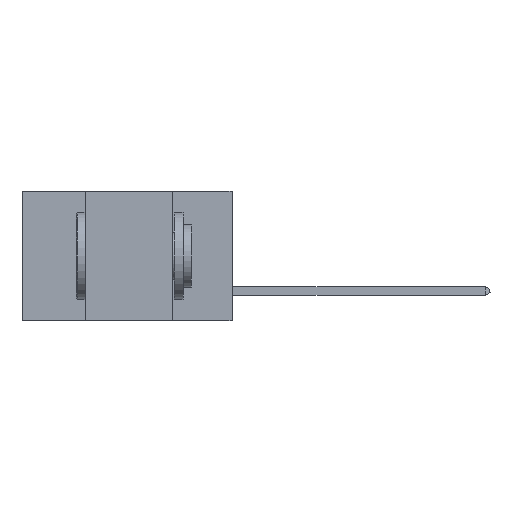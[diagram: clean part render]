
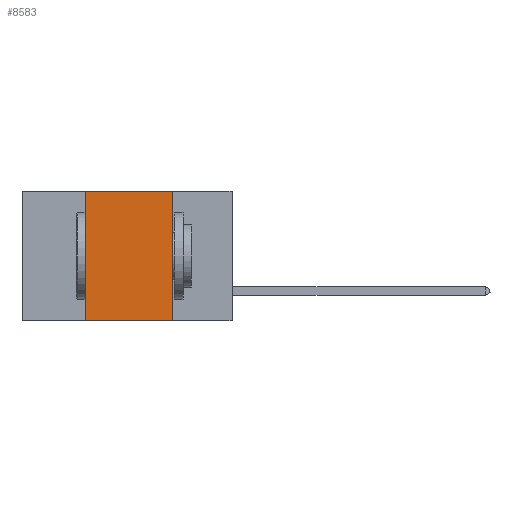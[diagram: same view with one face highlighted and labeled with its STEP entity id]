
A CAD part, left-side view. The second image highlights one B-rep face of the part: STEP entity #8583.
In plain terms, the highlighted planar face has unit normal (-1, 0, 0).
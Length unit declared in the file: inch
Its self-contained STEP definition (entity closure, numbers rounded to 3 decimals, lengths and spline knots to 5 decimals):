
#80 = ORIENTED_EDGE ( 'NONE', *, *, #19092, .T. ) ;
#405 = EDGE_LOOP ( 'NONE', ( #5363, #14550, #16608, #80 ) ) ;
#1328 = VECTOR ( 'NONE', #12689, 39.37008 ) ;
#1456 = CARTESIAN_POINT ( 'NONE',  ( 0., 0.6, 0. ) ) ;
#1559 = DIRECTION ( 'NONE',  ( 0., 0., -1. ) ) ;
#2734 = VERTEX_POINT ( 'NONE', #27336 ) ;
#5363 = ORIENTED_EDGE ( 'NONE', *, *, #26643, .F. ) ;
#6211 = VECTOR ( 'NONE', #12906, 39.37008 ) ;
#6416 = DIRECTION ( 'NONE',  ( 1., 0., 0. ) ) ;
#8298 = VERTEX_POINT ( 'NONE', #17225 ) ;
#8583 = ADVANCED_FACE ( 'NONE', ( #16068 ), #24759, .F. ) ;
#9105 = LINE ( 'NONE', #12541, #26764 ) ;
#10051 = VERTEX_POINT ( 'NONE', #23358 ) ;
#10774 = CARTESIAN_POINT ( 'NONE',  ( 0., 0.42, 0. ) ) ;
#12525 = LINE ( 'NONE', #24168, #1328 ) ;
#12541 = CARTESIAN_POINT ( 'NONE',  ( 0., 0.6, -0.37 ) ) ;
#12689 = DIRECTION ( 'NONE',  ( 0., 0., -1. ) ) ;
#12906 = DIRECTION ( 'NONE',  ( 0., 0., 1. ) ) ;
#13428 = DIRECTION ( 'NONE',  ( 0., -1., 0. ) ) ;
#14550 = ORIENTED_EDGE ( 'NONE', *, *, #28864, .F. ) ;
#16068 = FACE_OUTER_BOUND ( 'NONE', #405, .T. ) ;
#16608 = ORIENTED_EDGE ( 'NONE', *, *, #22581, .F. ) ;
#17225 = CARTESIAN_POINT ( 'NONE',  ( 0., 0.42, 0. ) ) ;
#17893 = VERTEX_POINT ( 'NONE', #22011 ) ;
#18553 = LINE ( 'NONE', #10774, #6211 ) ;
#18600 = VECTOR ( 'NONE', #13428, 39.37008 ) ;
#19092 = EDGE_CURVE ( 'NONE', #17893, #2734, #9105, .T. ) ;
#19309 = DIRECTION ( 'NONE',  ( 0., -1., 0. ) ) ;
#22011 = CARTESIAN_POINT ( 'NONE',  ( 0., 0.42, -0.37 ) ) ;
#22581 = EDGE_CURVE ( 'NONE', #17893, #8298, #18553, .T. ) ;
#22619 = CARTESIAN_POINT ( 'NONE',  ( 0., 0.6, 0. ) ) ;
#23358 = CARTESIAN_POINT ( 'NONE',  ( 0., 0.17, 0. ) ) ;
#24168 = CARTESIAN_POINT ( 'NONE',  ( 0., 0.17, 0. ) ) ;
#24759 = PLANE ( 'NONE',  #25352 ) ;
#25352 = AXIS2_PLACEMENT_3D ( 'NONE', #1456, #6416, #1559 ) ;
#26643 = EDGE_CURVE ( 'NONE', #10051, #2734, #12525, .T. ) ;
#26764 = VECTOR ( 'NONE', #19309, 39.37008 ) ;
#27336 = CARTESIAN_POINT ( 'NONE',  ( 0., 0.17, -0.37 ) ) ;
#28864 = EDGE_CURVE ( 'NONE', #8298, #10051, #29010, .T. ) ;
#29010 = LINE ( 'NONE', #22619, #18600 ) ;
